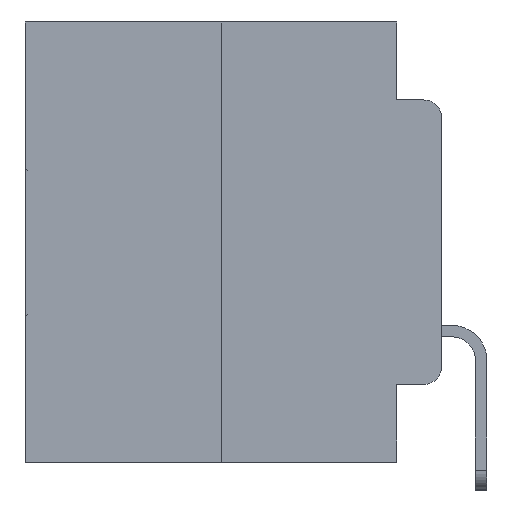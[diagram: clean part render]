
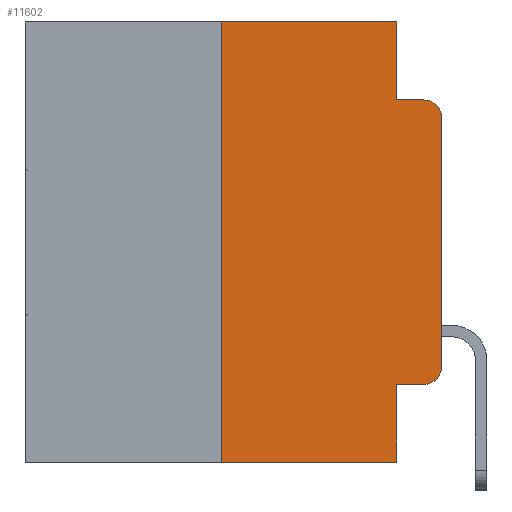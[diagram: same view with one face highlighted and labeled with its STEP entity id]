
A CAD part, left-side view. The second image highlights one B-rep face of the part: STEP entity #11602.
In plain terms, the highlighted planar face has unit normal (-1, 0, 0).
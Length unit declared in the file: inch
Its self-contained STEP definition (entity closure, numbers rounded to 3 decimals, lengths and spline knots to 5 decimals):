
#323 = LINE ( 'NONE', #14172, #7333 ) ;
#400 = EDGE_CURVE ( 'NONE', #3639, #28406, #7616, .T. ) ;
#706 = AXIS2_PLACEMENT_3D ( 'NONE', #6492, #21774, #8771 ) ;
#1122 = DIRECTION ( 'NONE',  ( -1., 0., 0. ) ) ;
#1146 = DIRECTION ( 'NONE',  ( 0., 0., -1. ) ) ;
#1235 = VECTOR ( 'NONE', #6479, 39.37008 ) ;
#1293 = CARTESIAN_POINT ( 'NONE',  ( 0., 0.02, -0.3915 ) ) ;
#1473 = CARTESIAN_POINT ( 'NONE',  ( 0., 0., 0. ) ) ;
#1605 = EDGE_CURVE ( 'NONE', #3537, #14685, #6835, .T. ) ;
#1973 = CARTESIAN_POINT ( 'NONE',  ( 0., 0.051, 0. ) ) ;
#2033 = EDGE_CURVE ( 'NONE', #28406, #12472, #2044, .T. ) ;
#2044 = CIRCLE ( 'NONE', #22975, 0.02 ) ;
#2266 = EDGE_CURVE ( 'NONE', #23143, #13719, #22809, .T. ) ;
#2296 = LINE ( 'NONE', #10098, #19445 ) ;
#2786 = DIRECTION ( 'NONE',  ( 0., -1., 0. ) ) ;
#3439 = CARTESIAN_POINT ( 'NONE',  ( 0., 0.473, 0. ) ) ;
#3537 = VERTEX_POINT ( 'NONE', #12835 ) ;
#3629 = ORIENTED_EDGE ( 'NONE', *, *, #400, .T. ) ;
#3639 = VERTEX_POINT ( 'NONE', #27671 ) ;
#3866 = DIRECTION ( 'NONE',  ( 0., 0., 1. ) ) ;
#4114 = ORIENTED_EDGE ( 'NONE', *, *, #2033, .T. ) ;
#4269 = ORIENTED_EDGE ( 'NONE', *, *, #19136, .F. ) ;
#5834 = CARTESIAN_POINT ( 'NONE',  ( 0., 0.25, 0. ) ) ;
#6479 = DIRECTION ( 'NONE',  ( 0., 0., 1. ) ) ;
#6492 = CARTESIAN_POINT ( 'NONE',  ( 0., 0.02, -0.1085 ) ) ;
#6689 = AXIS2_PLACEMENT_3D ( 'NONE', #3439, #12645, #27396 ) ;
#6835 = LINE ( 'NONE', #12389, #17956 ) ;
#7127 = ORIENTED_EDGE ( 'NONE', *, *, #1605, .T. ) ;
#7333 = VECTOR ( 'NONE', #2786, 39.37008 ) ;
#7616 = LINE ( 'NONE', #8511, #12927 ) ;
#8338 = ORIENTED_EDGE ( 'NONE', *, *, #20540, .T. ) ;
#8511 = CARTESIAN_POINT ( 'NONE',  ( 0., 0.051, -0.4115 ) ) ;
#8597 = DIRECTION ( 'NONE',  ( 0., -1., 0. ) ) ;
#8759 = CARTESIAN_POINT ( 'NONE',  ( 0., 0.25, 0. ) ) ;
#8771 = DIRECTION ( 'NONE',  ( 0., 0., -1. ) ) ;
#9353 = CARTESIAN_POINT ( 'NONE',  ( 0., 0., -0.3915 ) ) ;
#10098 = CARTESIAN_POINT ( 'NONE',  ( 0., 0.051, 0. ) ) ;
#10877 = ORIENTED_EDGE ( 'NONE', *, *, #14856, .F. ) ;
#11444 = VECTOR ( 'NONE', #19158, 39.37008 ) ;
#11474 = LINE ( 'NONE', #1473, #27672 ) ;
#11602 = ADVANCED_FACE ( 'NONE', ( #17047 ), #21159, .F. ) ;
#12129 = LINE ( 'NONE', #23309, #11444 ) ;
#12263 = CARTESIAN_POINT ( 'NONE',  ( 0., 0.051, -0.0885 ) ) ;
#12389 = CARTESIAN_POINT ( 'NONE',  ( 0., 0.473, -0.5 ) ) ;
#12472 = VERTEX_POINT ( 'NONE', #9353 ) ;
#12645 = DIRECTION ( 'NONE',  ( 1., 0., 0. ) ) ;
#12835 = CARTESIAN_POINT ( 'NONE',  ( 0., 0.25, -0.5 ) ) ;
#12927 = VECTOR ( 'NONE', #8597, 39.37008 ) ;
#13122 = ORIENTED_EDGE ( 'NONE', *, *, #24701, .F. ) ;
#13719 = VERTEX_POINT ( 'NONE', #1973 ) ;
#14172 = CARTESIAN_POINT ( 'NONE',  ( 0., 0.051, -0.0885 ) ) ;
#14685 = VERTEX_POINT ( 'NONE', #20803 ) ;
#14856 = EDGE_CURVE ( 'NONE', #13719, #26087, #12129, .T. ) ;
#15057 = CIRCLE ( 'NONE', #706, 0.02 ) ;
#17047 = FACE_OUTER_BOUND ( 'NONE', #18561, .T. ) ;
#17136 = CARTESIAN_POINT ( 'NONE',  ( 0., 0., -0.1085 ) ) ;
#17956 = VECTOR ( 'NONE', #24296, 39.37008 ) ;
#18442 = DIRECTION ( 'NONE',  ( 0., -1., 0. ) ) ;
#18481 = CARTESIAN_POINT ( 'NONE',  ( 0., 0.473, 0. ) ) ;
#18561 = EDGE_LOOP ( 'NONE', ( #25787, #8338, #4269, #10877, #24273, #13122, #7127, #25426, #3629, #4114 ) ) ;
#19136 = EDGE_CURVE ( 'NONE', #26087, #20633, #323, .T. ) ;
#19158 = DIRECTION ( 'NONE',  ( 0., 0., -1. ) ) ;
#19190 = LINE ( 'NONE', #8759, #1235 ) ;
#19445 = VECTOR ( 'NONE', #25039, 39.37008 ) ;
#20540 = EDGE_CURVE ( 'NONE', #28455, #20633, #15057, .T. ) ;
#20633 = VERTEX_POINT ( 'NONE', #28180 ) ;
#20803 = CARTESIAN_POINT ( 'NONE',  ( 0., 0.051, -0.5 ) ) ;
#21159 = PLANE ( 'NONE',  #6689 ) ;
#21774 = DIRECTION ( 'NONE',  ( -1., 0., 0. ) ) ;
#22181 = VECTOR ( 'NONE', #18442, 39.37008 ) ;
#22809 = LINE ( 'NONE', #18481, #22181 ) ;
#22975 = AXIS2_PLACEMENT_3D ( 'NONE', #1293, #1122, #1146 ) ;
#23143 = VERTEX_POINT ( 'NONE', #5834 ) ;
#23288 = EDGE_CURVE ( 'NONE', #12472, #28455, #11474, .T. ) ;
#23309 = CARTESIAN_POINT ( 'NONE',  ( 0., 0.051, 0. ) ) ;
#24273 = ORIENTED_EDGE ( 'NONE', *, *, #2266, .F. ) ;
#24296 = DIRECTION ( 'NONE',  ( 0., -1., 0. ) ) ;
#24701 = EDGE_CURVE ( 'NONE', #3537, #23143, #19190, .T. ) ;
#25039 = DIRECTION ( 'NONE',  ( 0., 0., -1. ) ) ;
#25327 = CARTESIAN_POINT ( 'NONE',  ( 0., 0.02, -0.4115 ) ) ;
#25426 = ORIENTED_EDGE ( 'NONE', *, *, #26095, .F. ) ;
#25787 = ORIENTED_EDGE ( 'NONE', *, *, #23288, .T. ) ;
#26087 = VERTEX_POINT ( 'NONE', #12263 ) ;
#26095 = EDGE_CURVE ( 'NONE', #3639, #14685, #2296, .T. ) ;
#27396 = DIRECTION ( 'NONE',  ( 0., 0., -1. ) ) ;
#27671 = CARTESIAN_POINT ( 'NONE',  ( 0., 0.051, -0.4115 ) ) ;
#27672 = VECTOR ( 'NONE', #3866, 39.37008 ) ;
#28180 = CARTESIAN_POINT ( 'NONE',  ( 0., 0.02, -0.0885 ) ) ;
#28406 = VERTEX_POINT ( 'NONE', #25327 ) ;
#28455 = VERTEX_POINT ( 'NONE', #17136 ) ;
